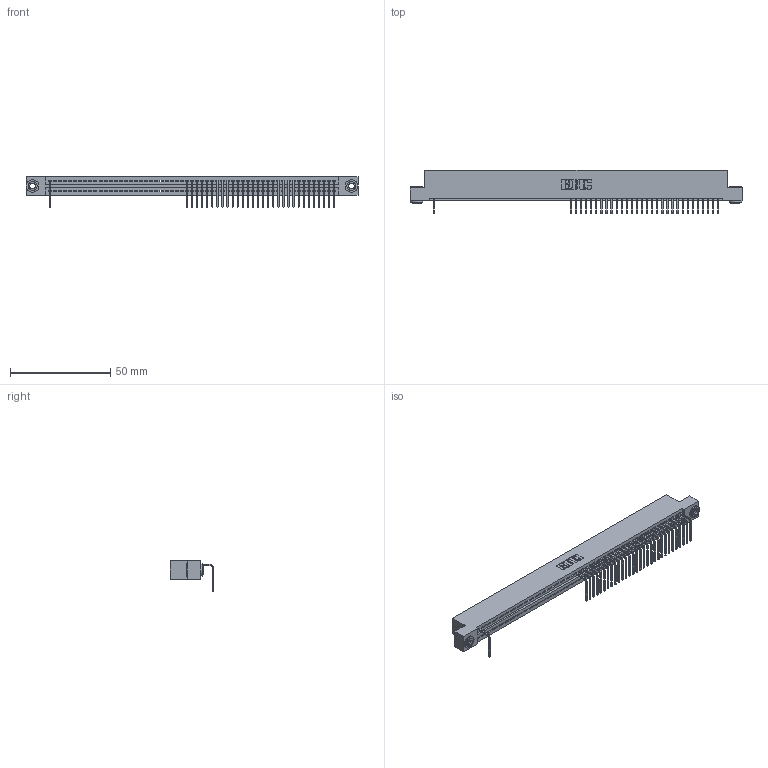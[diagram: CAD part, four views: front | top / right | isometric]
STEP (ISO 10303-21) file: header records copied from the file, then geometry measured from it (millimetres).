
FILE_DESCRIPTION (( 'STEP AP203' ), '1' );
FILE_NAME ('345-057-558-103.STEP', '2018-09-21T11:39:00', ( '' ), ( '' ), 'SwSTEP 2.0', 'SolidWorks 2016', '' );
FILE_SCHEMA (( 'CONFIG_CONTROL_DESIGN' ));
Length unit declared in the file: inch
Products named in the file (4): 345 Part_Flush Mounting Lugs - 0.156 Dia-TH; 345-292-001_558 Tail - 2; 345-250-002_345-250-002-102; 345-057-558-103
Assembly tree (34 placements, depth 2):
  345-057-558-103
    345 Part_Flush Mounting Lugs - 0.156 Dia-TH
    345-292-001_558 Tail - 2  x31
    345-250-002_345-250-002-102  x2
Bounding box: 165.99 x 21.83 x 15.37 mm (x, y, z)
Volume: 15713.6 mm3; surface area: 20326.2 mm2
Topology: 34 solids, 34 shells, 2440 faces, 7463 edges, 4930 vertices
Faces by surface type: plane 1756, cylinder 676, cone 8
Entity records: 40782 total; most frequent: ORIENTED_EDGE 7170, CARTESIAN_POINT 7160, DIRECTION 6233, EDGE_CURVE 3585, VECTOR 3201, LINE 3201, VERTEX_POINT 2386, AXIS2_PLACEMENT_3D 1516
